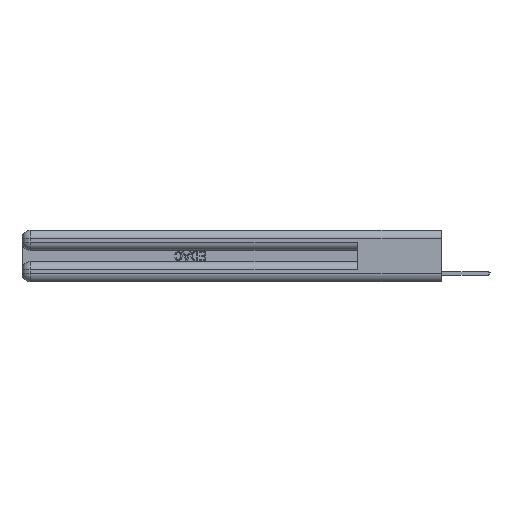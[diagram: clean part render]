
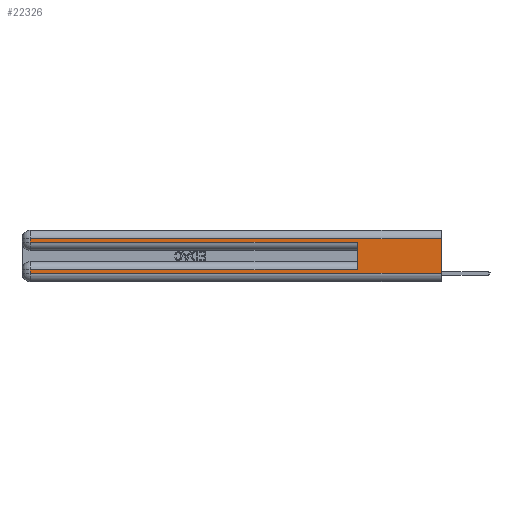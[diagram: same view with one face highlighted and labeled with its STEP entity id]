
A CAD part, left-side view. The second image highlights one B-rep face of the part: STEP entity #22326.
In plain terms, the highlighted planar face has unit normal (-1, 0, 0).
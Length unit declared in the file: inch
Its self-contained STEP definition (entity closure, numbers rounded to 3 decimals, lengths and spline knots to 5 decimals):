
#2 = LINE ( 'NONE', #29593, #26909 ) ;
#772 = VERTEX_POINT ( 'NONE', #20864 ) ;
#788 = DIRECTION ( 'NONE',  ( 0., -1., 0. ) ) ;
#884 = EDGE_CURVE ( 'NONE', #5710, #12632, #16692, .T. ) ;
#1841 = CARTESIAN_POINT ( 'NONE',  ( 0., 0.6, 0.285 ) ) ;
#1956 = ORIENTED_EDGE ( 'NONE', *, *, #4340, .T. ) ;
#2224 = CARTESIAN_POINT ( 'NONE',  ( 0., 0., 0.31 ) ) ;
#2492 = EDGE_CURVE ( 'NONE', #23105, #13956, #20302, .T. ) ;
#2815 = EDGE_CURVE ( 'NONE', #5856, #772, #14162, .T. ) ;
#3273 = PLANE ( 'NONE',  #9453 ) ;
#3866 = CARTESIAN_POINT ( 'NONE',  ( 0., 0.6, 0.085 ) ) ;
#4030 = CARTESIAN_POINT ( 'NONE',  ( 0., 0., 0.085 ) ) ;
#4340 = EDGE_CURVE ( 'NONE', #5710, #23105, #27072, .T. ) ;
#4519 = DIRECTION ( 'NONE',  ( 0., 1., 0. ) ) ;
#5710 = VERTEX_POINT ( 'NONE', #3866 ) ;
#5856 = VERTEX_POINT ( 'NONE', #16609 ) ;
#6869 = ORIENTED_EDGE ( 'NONE', *, *, #21851, .T. ) ;
#7235 = CARTESIAN_POINT ( 'NONE',  ( 0., 0., 0.285 ) ) ;
#7565 = CARTESIAN_POINT ( 'NONE',  ( 0., 0.6, 0.145 ) ) ;
#7876 = CARTESIAN_POINT ( 'NONE',  ( 0., 0., 0.06 ) ) ;
#8098 = DIRECTION ( 'NONE',  ( 1., 0., 0. ) ) ;
#9424 = DIRECTION ( 'NONE',  ( 0., 1., 0. ) ) ;
#9453 = AXIS2_PLACEMENT_3D ( 'NONE', #31715, #8098, #16153 ) ;
#10654 = VECTOR ( 'NONE', #14581, 39.37008 ) ;
#10849 = VECTOR ( 'NONE', #14938, 39.37008 ) ;
#11425 = VECTOR ( 'NONE', #26343, 39.37008 ) ;
#11763 = VECTOR ( 'NONE', #31499, 39.37008 ) ;
#12228 = ORIENTED_EDGE ( 'NONE', *, *, #2492, .T. ) ;
#12257 = ORIENTED_EDGE ( 'NONE', *, *, #18742, .T. ) ;
#12632 = VERTEX_POINT ( 'NONE', #1841 ) ;
#12744 = VECTOR ( 'NONE', #25221, 39.37008 ) ;
#13956 = VERTEX_POINT ( 'NONE', #26842 ) ;
#14162 = LINE ( 'NONE', #2224, #29211 ) ;
#14473 = ORIENTED_EDGE ( 'NONE', *, *, #17041, .T. ) ;
#14581 = DIRECTION ( 'NONE',  ( 0., 0., -1. ) ) ;
#14841 = VERTEX_POINT ( 'NONE', #27084 ) ;
#14938 = DIRECTION ( 'NONE',  ( 0., -1., 0. ) ) ;
#15925 = LINE ( 'NONE', #22376, #10654 ) ;
#16153 = DIRECTION ( 'NONE',  ( 0., 0., -1. ) ) ;
#16609 = CARTESIAN_POINT ( 'NONE',  ( 0., 0., 0.31 ) ) ;
#16692 = LINE ( 'NONE', #7565, #11425 ) ;
#17041 = EDGE_CURVE ( 'NONE', #772, #14841, #28244, .T. ) ;
#18545 = ORIENTED_EDGE ( 'NONE', *, *, #884, .F. ) ;
#18742 = EDGE_CURVE ( 'NONE', #14841, #12632, #21870, .T. ) ;
#20302 = LINE ( 'NONE', #28572, #11763 ) ;
#20864 = CARTESIAN_POINT ( 'NONE',  ( 0., 2.94, 0.31 ) ) ;
#21303 = EDGE_CURVE ( 'NONE', #5856, #31972, #15925, .T. ) ;
#21851 = EDGE_CURVE ( 'NONE', #13956, #31972, #2, .T. ) ;
#21870 = LINE ( 'NONE', #7235, #10849 ) ;
#22326 = ADVANCED_FACE ( 'NONE', ( #28884 ), #3273, .F. ) ;
#22376 = CARTESIAN_POINT ( 'NONE',  ( 0., 0., 0.37 ) ) ;
#23105 = VERTEX_POINT ( 'NONE', #24362 ) ;
#24362 = CARTESIAN_POINT ( 'NONE',  ( 0., 2.94, 0.085 ) ) ;
#24567 = CARTESIAN_POINT ( 'NONE',  ( 0., 2.94, 0.37 ) ) ;
#24795 = EDGE_LOOP ( 'NONE', ( #25421, #32583, #14473, #12257, #18545, #1956, #12228, #6869 ) ) ;
#25221 = DIRECTION ( 'NONE',  ( 0., 0., -1. ) ) ;
#25421 = ORIENTED_EDGE ( 'NONE', *, *, #21303, .F. ) ;
#26343 = DIRECTION ( 'NONE',  ( 0., 0., 1. ) ) ;
#26842 = CARTESIAN_POINT ( 'NONE',  ( 0., 2.94, 0.06 ) ) ;
#26909 = VECTOR ( 'NONE', #788, 39.37008 ) ;
#27072 = LINE ( 'NONE', #4030, #31127 ) ;
#27084 = CARTESIAN_POINT ( 'NONE',  ( 0., 2.94, 0.285 ) ) ;
#28244 = LINE ( 'NONE', #24567, #12744 ) ;
#28572 = CARTESIAN_POINT ( 'NONE',  ( 0., 2.94, 0.37 ) ) ;
#28884 = FACE_OUTER_BOUND ( 'NONE', #24795, .T. ) ;
#29211 = VECTOR ( 'NONE', #4519, 39.37008 ) ;
#29593 = CARTESIAN_POINT ( 'NONE',  ( 0., 0., 0.06 ) ) ;
#31127 = VECTOR ( 'NONE', #9424, 39.37008 ) ;
#31499 = DIRECTION ( 'NONE',  ( 0., 0., -1. ) ) ;
#31715 = CARTESIAN_POINT ( 'NONE',  ( 0., 0., 0.37 ) ) ;
#31972 = VERTEX_POINT ( 'NONE', #7876 ) ;
#32583 = ORIENTED_EDGE ( 'NONE', *, *, #2815, .T. ) ;
